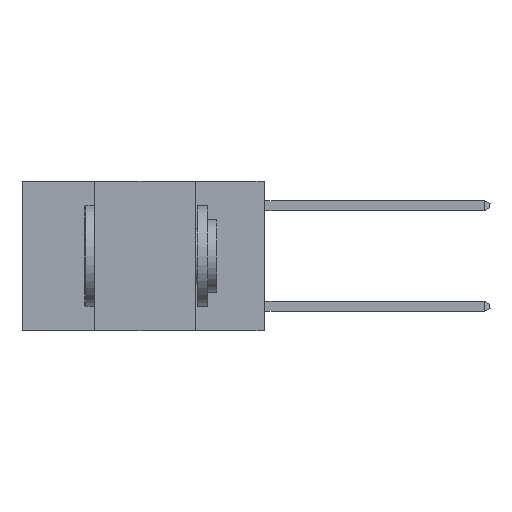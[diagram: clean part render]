
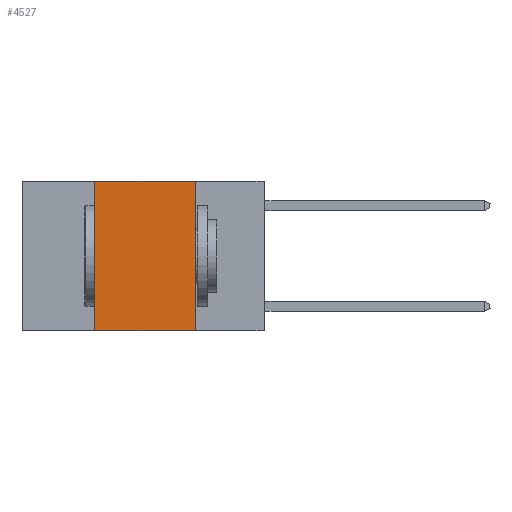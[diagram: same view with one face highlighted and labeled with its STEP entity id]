
A CAD part, left-side view. The second image highlights one B-rep face of the part: STEP entity #4527.
In plain terms, the highlighted planar face has unit normal (-1, 0, 0).
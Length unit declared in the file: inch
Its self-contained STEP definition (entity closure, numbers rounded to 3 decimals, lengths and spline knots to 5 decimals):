
#156 = DIRECTION ( 'NONE',  ( 0., 0., -1. ) ) ;
#524 = LINE ( 'NONE', #13837, #13663 ) ;
#745 = VERTEX_POINT ( 'NONE', #4149 ) ;
#1074 = VECTOR ( 'NONE', #5492, 39.37008 ) ;
#1489 = VECTOR ( 'NONE', #13928, 39.37008 ) ;
#2050 = DIRECTION ( 'NONE',  ( 0., -1., 0. ) ) ;
#2377 = CARTESIAN_POINT ( 'NONE',  ( 0., 0.42, 0. ) ) ;
#4149 = CARTESIAN_POINT ( 'NONE',  ( 0., 0.42, -0.37 ) ) ;
#4527 = ADVANCED_FACE ( 'NONE', ( #7253 ), #20857, .F. ) ;
#5253 = CARTESIAN_POINT ( 'NONE',  ( 0., 0.17, 0. ) ) ;
#5492 = DIRECTION ( 'NONE',  ( 0., 0., -1. ) ) ;
#6672 = LINE ( 'NONE', #21880, #21826 ) ;
#7010 = VERTEX_POINT ( 'NONE', #14383 ) ;
#7205 = EDGE_CURVE ( 'NONE', #745, #21279, #524, .T. ) ;
#7253 = FACE_OUTER_BOUND ( 'NONE', #12785, .T. ) ;
#7499 = CARTESIAN_POINT ( 'NONE',  ( 0., 0.6, 0. ) ) ;
#7993 = CARTESIAN_POINT ( 'NONE',  ( 0., 0.17, 0. ) ) ;
#8255 = ORIENTED_EDGE ( 'NONE', *, *, #7205, .T. ) ;
#8668 = EDGE_CURVE ( 'NONE', #7010, #13942, #6672, .T. ) ;
#9108 = LINE ( 'NONE', #5253, #1074 ) ;
#9279 = ORIENTED_EDGE ( 'NONE', *, *, #18049, .F. ) ;
#10017 = ORIENTED_EDGE ( 'NONE', *, *, #8668, .F. ) ;
#11322 = DIRECTION ( 'NONE',  ( 1., 0., 0. ) ) ;
#12132 = DIRECTION ( 'NONE',  ( 0., -1., 0. ) ) ;
#12785 = EDGE_LOOP ( 'NONE', ( #18176, #10017, #9279, #8255 ) ) ;
#13663 = VECTOR ( 'NONE', #2050, 39.37008 ) ;
#13837 = CARTESIAN_POINT ( 'NONE',  ( 0., 0.6, -0.37 ) ) ;
#13928 = DIRECTION ( 'NONE',  ( 0., 0., 1. ) ) ;
#13942 = VERTEX_POINT ( 'NONE', #7993 ) ;
#14383 = CARTESIAN_POINT ( 'NONE',  ( 0., 0.42, 0. ) ) ;
#15924 = AXIS2_PLACEMENT_3D ( 'NONE', #7499, #11322, #156 ) ;
#18049 = EDGE_CURVE ( 'NONE', #745, #7010, #22818, .T. ) ;
#18176 = ORIENTED_EDGE ( 'NONE', *, *, #21840, .F. ) ;
#18224 = CARTESIAN_POINT ( 'NONE',  ( 0., 0.17, -0.37 ) ) ;
#20857 = PLANE ( 'NONE',  #15924 ) ;
#21279 = VERTEX_POINT ( 'NONE', #18224 ) ;
#21826 = VECTOR ( 'NONE', #12132, 39.37008 ) ;
#21840 = EDGE_CURVE ( 'NONE', #13942, #21279, #9108, .T. ) ;
#21880 = CARTESIAN_POINT ( 'NONE',  ( 0., 0.6, 0. ) ) ;
#22818 = LINE ( 'NONE', #2377, #1489 ) ;
